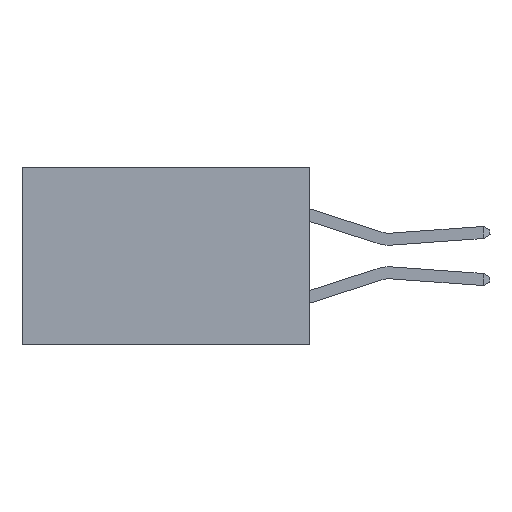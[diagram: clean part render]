
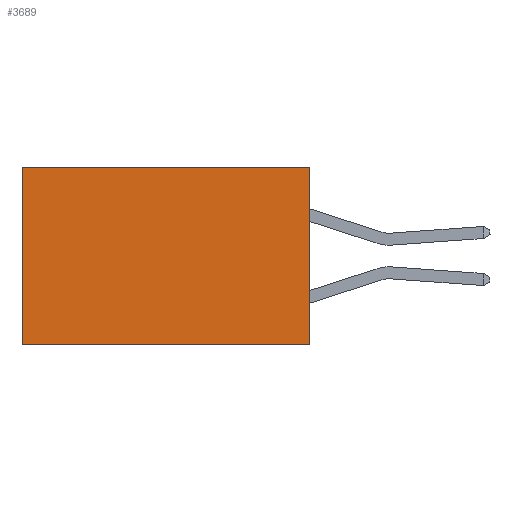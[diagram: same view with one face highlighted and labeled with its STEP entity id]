
A CAD part, left-side view. The second image highlights one B-rep face of the part: STEP entity #3689.
In plain terms, the highlighted planar face has unit normal (-1, 0, 0).
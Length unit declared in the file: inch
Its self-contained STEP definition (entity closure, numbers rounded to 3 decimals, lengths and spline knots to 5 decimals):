
#415 = LINE ( 'NONE', #7917, #6319 ) ;
#1059 = CARTESIAN_POINT ( 'NONE',  ( 0.2615, 0., -0.37 ) ) ;
#1300 = EDGE_CURVE ( 'NONE', #1948, #2130, #21736, .T. ) ;
#1856 = AXIS2_PLACEMENT_3D ( 'NONE', #7162, #14673, #10958 ) ;
#1948 = VERTEX_POINT ( 'NONE', #12727 ) ;
#2130 = VERTEX_POINT ( 'NONE', #20475 ) ;
#2817 = ORIENTED_EDGE ( 'NONE', *, *, #15677, .F. ) ;
#3689 = ADVANCED_FACE ( 'NONE', ( #18340 ), #22170, .F. ) ;
#4005 = EDGE_LOOP ( 'NONE', ( #13530, #2817, #22847, #17426 ) ) ;
#6319 = VECTOR ( 'NONE', #8031, 39.37008 ) ;
#7162 = CARTESIAN_POINT ( 'NONE',  ( 0.2615, 0., -0.37 ) ) ;
#7917 = CARTESIAN_POINT ( 'NONE',  ( 0.2615, 0.6, -0.37 ) ) ;
#8031 = DIRECTION ( 'NONE',  ( 0., 0., -1. ) ) ;
#8943 = DIRECTION ( 'NONE',  ( 0., 0., -1. ) ) ;
#8980 = VERTEX_POINT ( 'NONE', #21529 ) ;
#9855 = VECTOR ( 'NONE', #8943, 39.37008 ) ;
#10958 = DIRECTION ( 'NONE',  ( 0., 0., -1. ) ) ;
#12137 = VECTOR ( 'NONE', #19852, 39.37008 ) ;
#12243 = CARTESIAN_POINT ( 'NONE',  ( 0.2615, 0., -0.37 ) ) ;
#12727 = CARTESIAN_POINT ( 'NONE',  ( 0.2615, 0., 0. ) ) ;
#13530 = ORIENTED_EDGE ( 'NONE', *, *, #22160, .T. ) ;
#13805 = VECTOR ( 'NONE', #23565, 39.37008 ) ;
#13980 = CARTESIAN_POINT ( 'NONE',  ( 0.2615, 0., 0. ) ) ;
#14673 = DIRECTION ( 'NONE',  ( 1., 0., 0. ) ) ;
#15677 = EDGE_CURVE ( 'NONE', #15784, #8980, #19604, .T. ) ;
#15784 = VERTEX_POINT ( 'NONE', #12243 ) ;
#17426 = ORIENTED_EDGE ( 'NONE', *, *, #1300, .T. ) ;
#17918 = LINE ( 'NONE', #1059, #9855 ) ;
#18340 = FACE_OUTER_BOUND ( 'NONE', #4005, .T. ) ;
#18341 = EDGE_CURVE ( 'NONE', #1948, #15784, #17918, .T. ) ;
#19604 = LINE ( 'NONE', #23315, #12137 ) ;
#19852 = DIRECTION ( 'NONE',  ( 0., 1., 0. ) ) ;
#20475 = CARTESIAN_POINT ( 'NONE',  ( 0.2615, 0.6, 0. ) ) ;
#21529 = CARTESIAN_POINT ( 'NONE',  ( 0.2615, 0.6, -0.37 ) ) ;
#21736 = LINE ( 'NONE', #13980, #13805 ) ;
#22160 = EDGE_CURVE ( 'NONE', #2130, #8980, #415, .T. ) ;
#22170 = PLANE ( 'NONE',  #1856 ) ;
#22847 = ORIENTED_EDGE ( 'NONE', *, *, #18341, .F. ) ;
#23315 = CARTESIAN_POINT ( 'NONE',  ( 0.2615, 0., -0.37 ) ) ;
#23565 = DIRECTION ( 'NONE',  ( 0., 1., 0. ) ) ;
